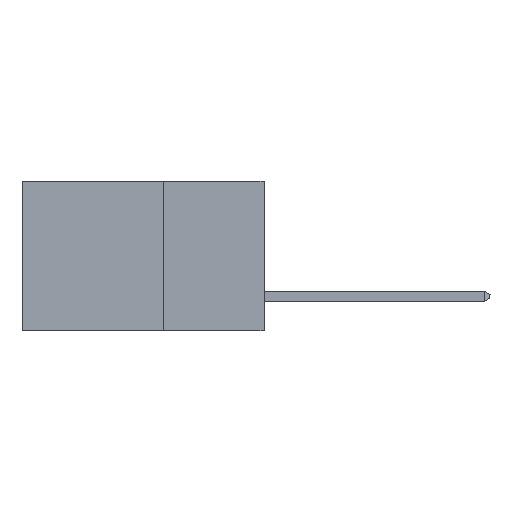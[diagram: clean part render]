
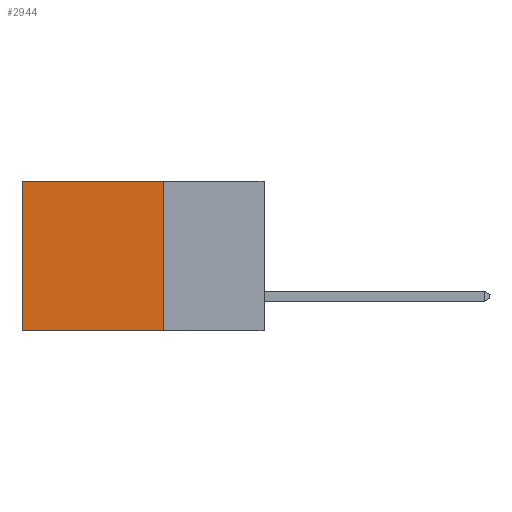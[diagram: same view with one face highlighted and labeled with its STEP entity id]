
A CAD part, left-side view. The second image highlights one B-rep face of the part: STEP entity #2944.
In plain terms, the highlighted planar face has unit normal (-1, 0, 0).
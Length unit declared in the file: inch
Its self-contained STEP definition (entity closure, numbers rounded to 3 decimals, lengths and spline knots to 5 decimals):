
#427 = PLANE ( 'NONE',  #22302 ) ;
#903 = VERTEX_POINT ( 'NONE', #23232 ) ;
#2022 = VECTOR ( 'NONE', #15310, 39.37008 ) ;
#2125 = LINE ( 'NONE', #10715, #20280 ) ;
#2297 = EDGE_LOOP ( 'NONE', ( #7935, #5486, #20222, #6551 ) ) ;
#2339 = VECTOR ( 'NONE', #23275, 39.37008 ) ;
#2944 = ADVANCED_FACE ( 'NONE', ( #16572 ), #427, .F. ) ;
#3071 = LINE ( 'NONE', #12135, #4616 ) ;
#3138 = DIRECTION ( 'NONE',  ( 0., 0., -1. ) ) ;
#3541 = EDGE_CURVE ( 'NONE', #15031, #8180, #2125, .T. ) ;
#4377 = EDGE_CURVE ( 'NONE', #5045, #903, #3071, .T. ) ;
#4616 = VECTOR ( 'NONE', #19338, 39.37008 ) ;
#5045 = VERTEX_POINT ( 'NONE', #19120 ) ;
#5486 = ORIENTED_EDGE ( 'NONE', *, *, #6415, .F. ) ;
#6415 = EDGE_CURVE ( 'NONE', #8180, #903, #8634, .T. ) ;
#6551 = ORIENTED_EDGE ( 'NONE', *, *, #10152, .T. ) ;
#7406 = DIRECTION ( 'NONE',  ( 0., 0., -1. ) ) ;
#7625 = CARTESIAN_POINT ( 'NONE',  ( 0.2615, 0.25, -0.37 ) ) ;
#7935 = ORIENTED_EDGE ( 'NONE', *, *, #4377, .T. ) ;
#8180 = VERTEX_POINT ( 'NONE', #19726 ) ;
#8634 = LINE ( 'NONE', #19377, #2339 ) ;
#10152 = EDGE_CURVE ( 'NONE', #15031, #5045, #16971, .T. ) ;
#10715 = CARTESIAN_POINT ( 'NONE',  ( 0.2615, 0.25, -0.37 ) ) ;
#12135 = CARTESIAN_POINT ( 'NONE',  ( 0.2615, 0.6, -0.37 ) ) ;
#14795 = DIRECTION ( 'NONE',  ( 1., 0., 0. ) ) ;
#15031 = VERTEX_POINT ( 'NONE', #15971 ) ;
#15310 = DIRECTION ( 'NONE',  ( 0., 1., 0. ) ) ;
#15971 = CARTESIAN_POINT ( 'NONE',  ( 0.2615, 0.25, 0. ) ) ;
#16572 = FACE_OUTER_BOUND ( 'NONE', #2297, .T. ) ;
#16971 = LINE ( 'NONE', #17080, #2022 ) ;
#17080 = CARTESIAN_POINT ( 'NONE',  ( 0.2615, 0.25, 0. ) ) ;
#19120 = CARTESIAN_POINT ( 'NONE',  ( 0.2615, 0.6, 0. ) ) ;
#19338 = DIRECTION ( 'NONE',  ( 0., 0., -1. ) ) ;
#19377 = CARTESIAN_POINT ( 'NONE',  ( 0.2615, 0.25, -0.37 ) ) ;
#19726 = CARTESIAN_POINT ( 'NONE',  ( 0.2615, 0.25, -0.37 ) ) ;
#20222 = ORIENTED_EDGE ( 'NONE', *, *, #3541, .F. ) ;
#20280 = VECTOR ( 'NONE', #7406, 39.37008 ) ;
#22302 = AXIS2_PLACEMENT_3D ( 'NONE', #7625, #14795, #3138 ) ;
#23232 = CARTESIAN_POINT ( 'NONE',  ( 0.2615, 0.6, -0.37 ) ) ;
#23275 = DIRECTION ( 'NONE',  ( 0., 1., 0. ) ) ;
